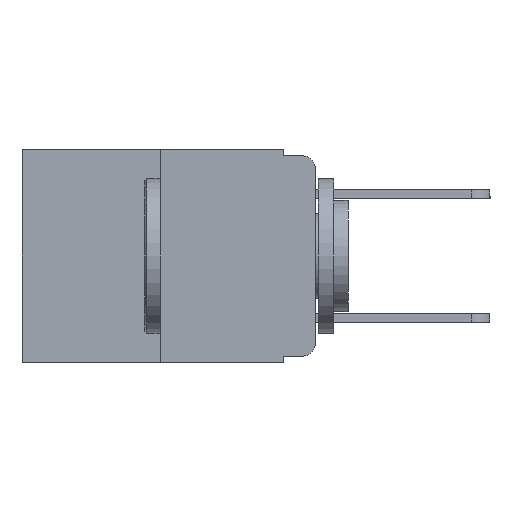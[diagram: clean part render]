
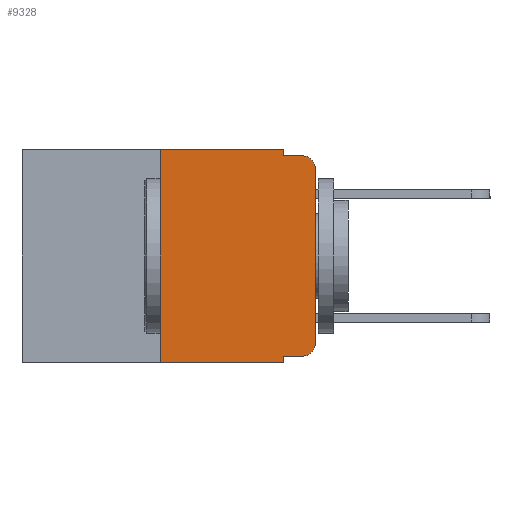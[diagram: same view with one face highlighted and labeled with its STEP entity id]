
A CAD part, left-side view. The second image highlights one B-rep face of the part: STEP entity #9328.
In plain terms, the highlighted planar face has unit normal (-1, 0, 0).
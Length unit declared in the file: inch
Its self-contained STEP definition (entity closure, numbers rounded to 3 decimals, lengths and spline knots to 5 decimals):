
#340 = LINE ( 'NONE', #17761, #4454 ) ;
#366 = CARTESIAN_POINT ( 'NONE',  ( 0., 0.051, 0. ) ) ;
#727 = CARTESIAN_POINT ( 'NONE',  ( 0., 0., -0.03 ) ) ;
#948 = CARTESIAN_POINT ( 'NONE',  ( 0., 0.473, 0. ) ) ;
#1394 = CARTESIAN_POINT ( 'NONE',  ( 0., 0.473, -0.343 ) ) ;
#1559 = CARTESIAN_POINT ( 'NONE',  ( 0., 0.02, -0.03 ) ) ;
#1782 = CARTESIAN_POINT ( 'NONE',  ( 0., 0.051, -0.01 ) ) ;
#2323 = EDGE_CURVE ( 'NONE', #8150, #6776, #5013, .T. ) ;
#2331 = CARTESIAN_POINT ( 'NONE',  ( 0., 0.25, -0.343 ) ) ;
#3107 = CARTESIAN_POINT ( 'NONE',  ( 0., 0.02, -0.313 ) ) ;
#3308 = DIRECTION ( 'NONE',  ( 0., 0., -1. ) ) ;
#3348 = LINE ( 'NONE', #948, #17383 ) ;
#3898 = DIRECTION ( 'NONE',  ( 0., 0., -1. ) ) ;
#4454 = VECTOR ( 'NONE', #16172, 39.37008 ) ;
#4817 = CARTESIAN_POINT ( 'NONE',  ( 0., 0.473, 0. ) ) ;
#4879 = DIRECTION ( 'NONE',  ( 0., 0., -1. ) ) ;
#4925 = DIRECTION ( 'NONE',  ( 0., -1., 0. ) ) ;
#5013 = LINE ( 'NONE', #7491, #9684 ) ;
#5151 = EDGE_CURVE ( 'NONE', #10211, #16718, #3348, .T. ) ;
#5337 = ORIENTED_EDGE ( 'NONE', *, *, #22011, .F. ) ;
#5392 = DIRECTION ( 'NONE',  ( 0., -1., 0. ) ) ;
#5670 = VERTEX_POINT ( 'NONE', #7532 ) ;
#5703 = AXIS2_PLACEMENT_3D ( 'NONE', #3107, #15440, #4879 ) ;
#5864 = ORIENTED_EDGE ( 'NONE', *, *, #10223, .F. ) ;
#6187 = VERTEX_POINT ( 'NONE', #14229 ) ;
#6577 = DIRECTION ( 'NONE',  ( 0., 0., -1. ) ) ;
#6776 = VERTEX_POINT ( 'NONE', #12430 ) ;
#6892 = AXIS2_PLACEMENT_3D ( 'NONE', #4817, #17113, #6577 ) ;
#6930 = LINE ( 'NONE', #9790, #20278 ) ;
#7491 = CARTESIAN_POINT ( 'NONE',  ( 0., 0.051, 0. ) ) ;
#7532 = CARTESIAN_POINT ( 'NONE',  ( 0., 0.02, -0.333 ) ) ;
#8150 = VERTEX_POINT ( 'NONE', #20836 ) ;
#8321 = DIRECTION ( 'NONE',  ( 0., 0., -1. ) ) ;
#8648 = ORIENTED_EDGE ( 'NONE', *, *, #10020, .T. ) ;
#9096 = VECTOR ( 'NONE', #5392, 39.37008 ) ;
#9148 = CARTESIAN_POINT ( 'NONE',  ( 0., 0.25, 0. ) ) ;
#9328 = ADVANCED_FACE ( 'NONE', ( #13381 ), #15296, .F. ) ;
#9347 = EDGE_CURVE ( 'NONE', #5670, #6187, #18014, .T. ) ;
#9684 = VECTOR ( 'NONE', #8321, 39.37008 ) ;
#9723 = DIRECTION ( 'NONE',  ( 0., 0., 1. ) ) ;
#9790 = CARTESIAN_POINT ( 'NONE',  ( 0., 0.25, 0. ) ) ;
#10014 = ORIENTED_EDGE ( 'NONE', *, *, #13846, .T. ) ;
#10020 = EDGE_CURVE ( 'NONE', #15622, #6776, #22299, .T. ) ;
#10030 = ORIENTED_EDGE ( 'NONE', *, *, #16855, .T. ) ;
#10061 = EDGE_CURVE ( 'NONE', #17735, #21793, #13079, .T. ) ;
#10211 = VERTEX_POINT ( 'NONE', #9148 ) ;
#10223 = EDGE_CURVE ( 'NONE', #16718, #18694, #18620, .T. ) ;
#11129 = CARTESIAN_POINT ( 'NONE',  ( 0., 0., 0. ) ) ;
#11418 = ORIENTED_EDGE ( 'NONE', *, *, #2323, .F. ) ;
#12430 = CARTESIAN_POINT ( 'NONE',  ( 0., 0.051, -0.343 ) ) ;
#12766 = VECTOR ( 'NONE', #9723, 39.37008 ) ;
#13079 = CIRCLE ( 'NONE', #14270, 0.02 ) ;
#13381 = FACE_OUTER_BOUND ( 'NONE', #21913, .T. ) ;
#13791 = CARTESIAN_POINT ( 'NONE',  ( 0., 0.051, 0. ) ) ;
#13793 = LINE ( 'NONE', #15927, #9096 ) ;
#13846 = EDGE_CURVE ( 'NONE', #6187, #17735, #21976, .T. ) ;
#13895 = DIRECTION ( 'NONE',  ( -1., 0., 0. ) ) ;
#14224 = EDGE_CURVE ( 'NONE', #18694, #21793, #340, .T. ) ;
#14229 = CARTESIAN_POINT ( 'NONE',  ( 0., 0., -0.313 ) ) ;
#14270 = AXIS2_PLACEMENT_3D ( 'NONE', #1559, #13895, #3308 ) ;
#15296 = PLANE ( 'NONE',  #6892 ) ;
#15440 = DIRECTION ( 'NONE',  ( -1., 0., 0. ) ) ;
#15622 = VERTEX_POINT ( 'NONE', #2331 ) ;
#15927 = CARTESIAN_POINT ( 'NONE',  ( 0., 0.051, -0.333 ) ) ;
#16172 = DIRECTION ( 'NONE',  ( 0., -1., 0. ) ) ;
#16580 = ORIENTED_EDGE ( 'NONE', *, *, #14224, .F. ) ;
#16718 = VERTEX_POINT ( 'NONE', #13791 ) ;
#16855 = EDGE_CURVE ( 'NONE', #8150, #5670, #13793, .T. ) ;
#17113 = DIRECTION ( 'NONE',  ( 1., 0., 0. ) ) ;
#17383 = VECTOR ( 'NONE', #21956, 39.37008 ) ;
#17725 = VECTOR ( 'NONE', #4925, 39.37008 ) ;
#17735 = VERTEX_POINT ( 'NONE', #727 ) ;
#17761 = CARTESIAN_POINT ( 'NONE',  ( 0., 0.051, -0.01 ) ) ;
#18014 = CIRCLE ( 'NONE', #5703, 0.02 ) ;
#18100 = VECTOR ( 'NONE', #3898, 39.37008 ) ;
#18440 = ORIENTED_EDGE ( 'NONE', *, *, #10061, .T. ) ;
#18506 = ORIENTED_EDGE ( 'NONE', *, *, #9347, .T. ) ;
#18620 = LINE ( 'NONE', #366, #18100 ) ;
#18694 = VERTEX_POINT ( 'NONE', #1782 ) ;
#19456 = CARTESIAN_POINT ( 'NONE',  ( 0., 0.02, -0.01 ) ) ;
#20278 = VECTOR ( 'NONE', #22047, 39.37008 ) ;
#20620 = ORIENTED_EDGE ( 'NONE', *, *, #5151, .F. ) ;
#20836 = CARTESIAN_POINT ( 'NONE',  ( 0., 0.051, -0.333 ) ) ;
#21793 = VERTEX_POINT ( 'NONE', #19456 ) ;
#21913 = EDGE_LOOP ( 'NONE', ( #10014, #18440, #16580, #5864, #20620, #5337, #8648, #11418, #10030, #18506 ) ) ;
#21956 = DIRECTION ( 'NONE',  ( 0., -1., 0. ) ) ;
#21976 = LINE ( 'NONE', #11129, #12766 ) ;
#22011 = EDGE_CURVE ( 'NONE', #15622, #10211, #6930, .T. ) ;
#22047 = DIRECTION ( 'NONE',  ( 0., 0., 1. ) ) ;
#22299 = LINE ( 'NONE', #1394, #17725 ) ;
